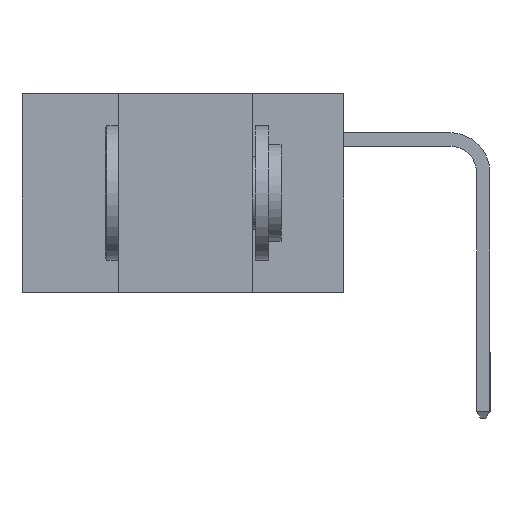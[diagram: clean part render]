
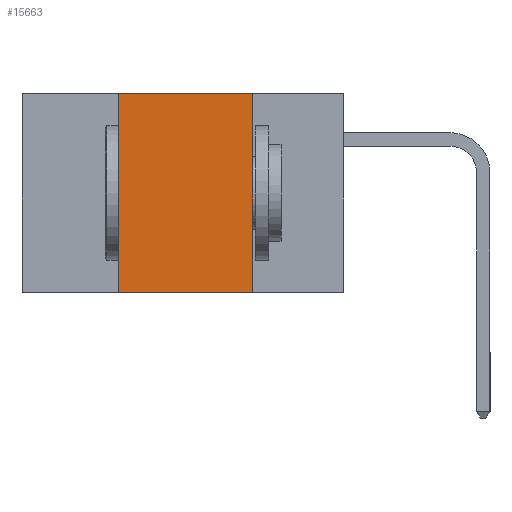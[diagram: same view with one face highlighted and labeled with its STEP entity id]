
A CAD part, left-side view. The second image highlights one B-rep face of the part: STEP entity #15663.
In plain terms, the highlighted planar face has unit normal (-1, 0, 0).
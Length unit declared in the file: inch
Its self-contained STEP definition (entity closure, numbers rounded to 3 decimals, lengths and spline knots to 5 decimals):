
#652 = EDGE_CURVE ( 'NONE', #10732, #23960, #17866, .T. ) ;
#1007 = CARTESIAN_POINT ( 'NONE',  ( 0., 0.6, 0. ) ) ;
#1218 = VECTOR ( 'NONE', #11888, 39.37008 ) ;
#3350 = DIRECTION ( 'NONE',  ( 0., -1., 0. ) ) ;
#3443 = ORIENTED_EDGE ( 'NONE', *, *, #14060, .F. ) ;
#4683 = VECTOR ( 'NONE', #14291, 39.37008 ) ;
#5252 = ORIENTED_EDGE ( 'NONE', *, *, #12984, .F. ) ;
#5602 = CARTESIAN_POINT ( 'NONE',  ( 0., 0.42, 0. ) ) ;
#6189 = VECTOR ( 'NONE', #19989, 39.37008 ) ;
#6685 = CARTESIAN_POINT ( 'NONE',  ( 0., 0.17, 0. ) ) ;
#6743 = VERTEX_POINT ( 'NONE', #17260 ) ;
#6758 = VECTOR ( 'NONE', #3350, 39.37008 ) ;
#6907 = EDGE_LOOP ( 'NONE', ( #5252, #3443, #17756, #23984 ) ) ;
#7361 = LINE ( 'NONE', #18377, #6758 ) ;
#7640 = VERTEX_POINT ( 'NONE', #7992 ) ;
#7992 = CARTESIAN_POINT ( 'NONE',  ( 0., 0.17, 0. ) ) ;
#10732 = VERTEX_POINT ( 'NONE', #11944 ) ;
#11888 = DIRECTION ( 'NONE',  ( 0., 0., 1. ) ) ;
#11944 = CARTESIAN_POINT ( 'NONE',  ( 0., 0.42, -0.37 ) ) ;
#12143 = DIRECTION ( 'NONE',  ( 0., 0., -1. ) ) ;
#12220 = FACE_OUTER_BOUND ( 'NONE', #6907, .T. ) ;
#12984 = EDGE_CURVE ( 'NONE', #7640, #6743, #16272, .T. ) ;
#13713 = PLANE ( 'NONE',  #16156 ) ;
#14060 = EDGE_CURVE ( 'NONE', #23960, #7640, #22563, .T. ) ;
#14291 = DIRECTION ( 'NONE',  ( 0., -1., 0. ) ) ;
#15663 = ADVANCED_FACE ( 'NONE', ( #12220 ), #13713, .F. ) ;
#15863 = DIRECTION ( 'NONE',  ( 1., 0., 0. ) ) ;
#16156 = AXIS2_PLACEMENT_3D ( 'NONE', #23519, #15863, #12143 ) ;
#16272 = LINE ( 'NONE', #6685, #6189 ) ;
#17260 = CARTESIAN_POINT ( 'NONE',  ( 0., 0.17, -0.37 ) ) ;
#17756 = ORIENTED_EDGE ( 'NONE', *, *, #652, .F. ) ;
#17866 = LINE ( 'NONE', #23276, #1218 ) ;
#18377 = CARTESIAN_POINT ( 'NONE',  ( 0., 0.6, -0.37 ) ) ;
#19249 = EDGE_CURVE ( 'NONE', #10732, #6743, #7361, .T. ) ;
#19989 = DIRECTION ( 'NONE',  ( 0., 0., -1. ) ) ;
#22563 = LINE ( 'NONE', #1007, #4683 ) ;
#23276 = CARTESIAN_POINT ( 'NONE',  ( 0., 0.42, 0. ) ) ;
#23519 = CARTESIAN_POINT ( 'NONE',  ( 0., 0.6, 0. ) ) ;
#23960 = VERTEX_POINT ( 'NONE', #5602 ) ;
#23984 = ORIENTED_EDGE ( 'NONE', *, *, #19249, .T. ) ;
